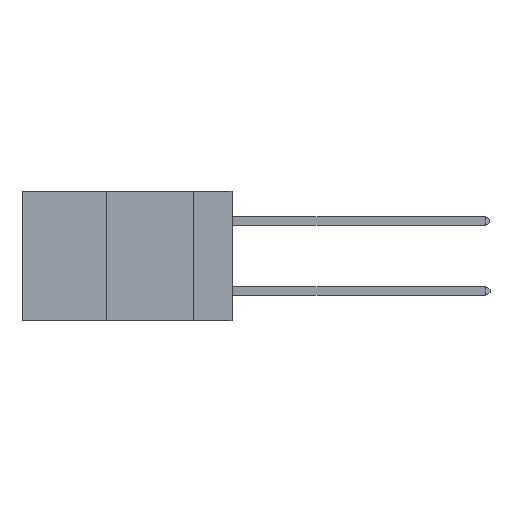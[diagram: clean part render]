
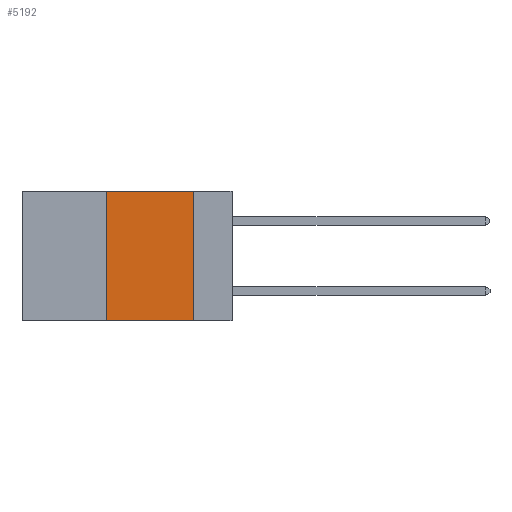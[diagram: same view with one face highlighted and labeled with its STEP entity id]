
A CAD part, left-side view. The second image highlights one B-rep face of the part: STEP entity #5192.
In plain terms, the highlighted planar face has unit normal (-1, 0, 0).
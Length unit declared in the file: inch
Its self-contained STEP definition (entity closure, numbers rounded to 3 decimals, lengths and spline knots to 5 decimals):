
#297 = LINE ( 'NONE', #12043, #14736 ) ;
#2194 = AXIS2_PLACEMENT_3D ( 'NONE', #9263, #5052, #14754 ) ;
#2292 = CARTESIAN_POINT ( 'NONE',  ( 0., 0.6, -0.37 ) ) ;
#2461 = EDGE_LOOP ( 'NONE', ( #9431, #6126, #13516, #13921 ) ) ;
#2713 = VECTOR ( 'NONE', #9349, 39.37008 ) ;
#3088 = VECTOR ( 'NONE', #4899, 39.37008 ) ;
#3132 = VERTEX_POINT ( 'NONE', #16624 ) ;
#3671 = PLANE ( 'NONE',  #2194 ) ;
#4303 = VECTOR ( 'NONE', #11490, 39.37008 ) ;
#4745 = FACE_OUTER_BOUND ( 'NONE', #2461, .T. ) ;
#4899 = DIRECTION ( 'NONE',  ( 0., -1., 0. ) ) ;
#5052 = DIRECTION ( 'NONE',  ( 1., 0., 0. ) ) ;
#5192 = ADVANCED_FACE ( 'NONE', ( #4745 ), #3671, .F. ) ;
#6126 = ORIENTED_EDGE ( 'NONE', *, *, #15064, .F. ) ;
#6827 = LINE ( 'NONE', #14631, #3088 ) ;
#6891 = LINE ( 'NONE', #2292, #2713 ) ;
#7268 = CARTESIAN_POINT ( 'NONE',  ( 0., 0.11, 0. ) ) ;
#8071 = LINE ( 'NONE', #7268, #4303 ) ;
#8805 = CARTESIAN_POINT ( 'NONE',  ( 0., 0.36, 0. ) ) ;
#9142 = DIRECTION ( 'NONE',  ( 0., 0., 1. ) ) ;
#9263 = CARTESIAN_POINT ( 'NONE',  ( 0., 0.6, 0. ) ) ;
#9349 = DIRECTION ( 'NONE',  ( 0., -1., 0. ) ) ;
#9431 = ORIENTED_EDGE ( 'NONE', *, *, #10627, .F. ) ;
#9590 = VERTEX_POINT ( 'NONE', #14594 ) ;
#10627 = EDGE_CURVE ( 'NONE', #9590, #13078, #8071, .T. ) ;
#11490 = DIRECTION ( 'NONE',  ( 0., 0., -1. ) ) ;
#11563 = EDGE_CURVE ( 'NONE', #3132, #13136, #297, .T. ) ;
#12043 = CARTESIAN_POINT ( 'NONE',  ( 0., 0.36, 0. ) ) ;
#12790 = CARTESIAN_POINT ( 'NONE',  ( 0., 0.11, -0.37 ) ) ;
#13078 = VERTEX_POINT ( 'NONE', #12790 ) ;
#13136 = VERTEX_POINT ( 'NONE', #8805 ) ;
#13378 = EDGE_CURVE ( 'NONE', #3132, #13078, #6891, .T. ) ;
#13516 = ORIENTED_EDGE ( 'NONE', *, *, #11563, .F. ) ;
#13921 = ORIENTED_EDGE ( 'NONE', *, *, #13378, .T. ) ;
#14594 = CARTESIAN_POINT ( 'NONE',  ( 0., 0.11, 0. ) ) ;
#14631 = CARTESIAN_POINT ( 'NONE',  ( 0., 0.6, 0. ) ) ;
#14736 = VECTOR ( 'NONE', #9142, 39.37008 ) ;
#14754 = DIRECTION ( 'NONE',  ( 0., 0., -1. ) ) ;
#15064 = EDGE_CURVE ( 'NONE', #13136, #9590, #6827, .T. ) ;
#16624 = CARTESIAN_POINT ( 'NONE',  ( 0., 0.36, -0.37 ) ) ;
